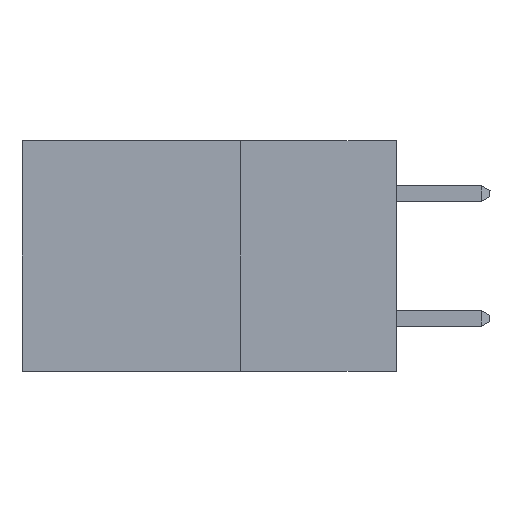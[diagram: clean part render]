
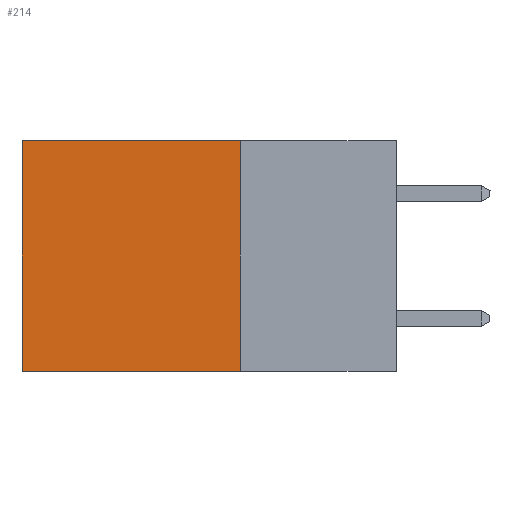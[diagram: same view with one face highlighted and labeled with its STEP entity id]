
A CAD part, left-side view. The second image highlights one B-rep face of the part: STEP entity #214.
In plain terms, the highlighted planar face has unit normal (-1, 0, 0).
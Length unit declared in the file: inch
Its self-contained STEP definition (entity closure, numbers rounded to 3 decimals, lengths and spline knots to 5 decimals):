
#214 = ADVANCED_FACE ( 'NONE', ( #7063 ), #6957, .F. ) ;
#480 = CARTESIAN_POINT ( 'NONE',  ( 0.298, 0.25, 0. ) ) ;
#588 = CARTESIAN_POINT ( 'NONE',  ( 0.298, 0.25, 0. ) ) ;
#1227 = VERTEX_POINT ( 'NONE', #7057 ) ;
#1619 = EDGE_LOOP ( 'NONE', ( #13300, #8415, #2133, #8167 ) ) ;
#2133 = ORIENTED_EDGE ( 'NONE', *, *, #7915, .F. ) ;
#3013 = AXIS2_PLACEMENT_3D ( 'NONE', #9308, #7402, #12258 ) ;
#3809 = DIRECTION ( 'NONE',  ( 0., 0., -1. ) ) ;
#4464 = CARTESIAN_POINT ( 'NONE',  ( 0.298, 0.25, -0.37 ) ) ;
#4665 = EDGE_CURVE ( 'NONE', #12098, #13566, #10780, .T. ) ;
#6680 = VECTOR ( 'NONE', #9207, 39.37008 ) ;
#6957 = PLANE ( 'NONE',  #3013 ) ;
#7043 = LINE ( 'NONE', #4464, #12227 ) ;
#7057 = CARTESIAN_POINT ( 'NONE',  ( 0.298, 0.25, -0.37 ) ) ;
#7063 = FACE_OUTER_BOUND ( 'NONE', #1619, .T. ) ;
#7402 = DIRECTION ( 'NONE',  ( 1., 0., 0. ) ) ;
#7915 = EDGE_CURVE ( 'NONE', #13412, #1227, #12292, .T. ) ;
#8167 = ORIENTED_EDGE ( 'NONE', *, *, #11517, .T. ) ;
#8415 = ORIENTED_EDGE ( 'NONE', *, *, #10021, .F. ) ;
#8436 = CARTESIAN_POINT ( 'NONE',  ( 0.298, 0.6, 0. ) ) ;
#9207 = DIRECTION ( 'NONE',  ( 0., 1., 0. ) ) ;
#9308 = CARTESIAN_POINT ( 'NONE',  ( 0.298, 0.25, 0. ) ) ;
#9495 = DIRECTION ( 'NONE',  ( 0., 0., -1. ) ) ;
#10021 = EDGE_CURVE ( 'NONE', #1227, #13566, #7043, .T. ) ;
#10341 = CARTESIAN_POINT ( 'NONE',  ( 0.298, 0.6, 0. ) ) ;
#10488 = CARTESIAN_POINT ( 'NONE',  ( 0.298, 0.25, 0. ) ) ;
#10780 = LINE ( 'NONE', #8436, #12540 ) ;
#10794 = DIRECTION ( 'NONE',  ( 0., 1., 0. ) ) ;
#11517 = EDGE_CURVE ( 'NONE', #13412, #12098, #12204, .T. ) ;
#11731 = CARTESIAN_POINT ( 'NONE',  ( 0.298, 0.6, -0.37 ) ) ;
#11958 = VECTOR ( 'NONE', #3809, 39.37008 ) ;
#12098 = VERTEX_POINT ( 'NONE', #10341 ) ;
#12204 = LINE ( 'NONE', #588, #6680 ) ;
#12227 = VECTOR ( 'NONE', #10794, 39.37008 ) ;
#12258 = DIRECTION ( 'NONE',  ( 0., 0., -1. ) ) ;
#12292 = LINE ( 'NONE', #480, #11958 ) ;
#12540 = VECTOR ( 'NONE', #9495, 39.37008 ) ;
#13300 = ORIENTED_EDGE ( 'NONE', *, *, #4665, .T. ) ;
#13412 = VERTEX_POINT ( 'NONE', #10488 ) ;
#13566 = VERTEX_POINT ( 'NONE', #11731 ) ;
